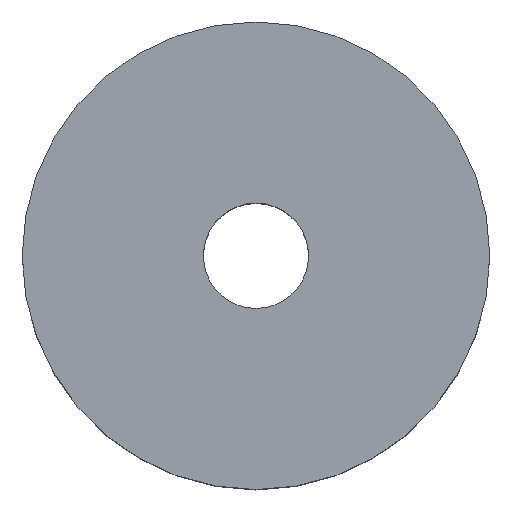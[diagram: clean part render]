
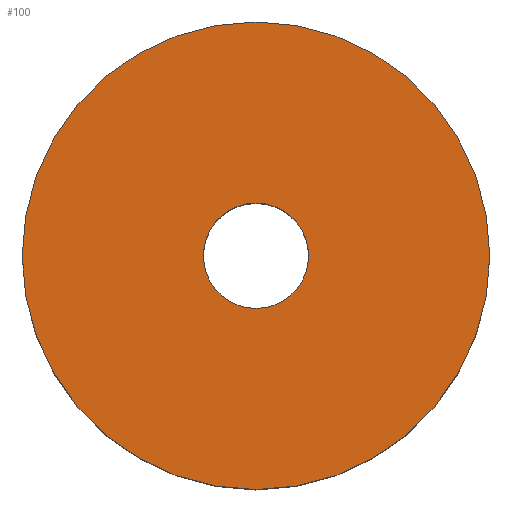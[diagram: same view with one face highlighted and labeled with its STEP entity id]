
A CAD part, top view. The second image highlights one B-rep face of the part: STEP entity #100.
In plain terms, the highlighted planar face has unit normal (0, 0, 1).
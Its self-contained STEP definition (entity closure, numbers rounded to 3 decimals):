
#5 = DIRECTION ( 'NONE',  ( 1., 0., 0. ) ) ;
#6 = DIRECTION ( 'NONE',  ( 0., 0., 1. ) ) ;
#7 = CARTESIAN_POINT ( 'NONE',  ( 0., 0., 5. ) ) ;
#12 = DIRECTION ( 'NONE',  ( 1., 0., 0. ) ) ;
#17 = VERTEX_POINT ( 'NONE', #87 ) ;
#21 = DIRECTION ( 'NONE',  ( 0., 0., 1. ) ) ;
#31 = CARTESIAN_POINT ( 'NONE',  ( 0., 0., 5. ) ) ;
#38 = CARTESIAN_POINT ( 'NONE',  ( -1.125, 0., 5. ) ) ;
#43 = CARTESIAN_POINT ( 'NONE',  ( 5., 0., 5. ) ) ;
#44 = CARTESIAN_POINT ( 'NONE',  ( -5., 0., 5. ) ) ;
#51 = DIRECTION ( 'NONE',  ( 1., 0., 0. ) ) ;
#53 = DIRECTION ( 'NONE',  ( 1., 0., 0. ) ) ;
#55 = PLANE ( 'NONE',  #179 ) ;
#59 = DIRECTION ( 'NONE',  ( 0., 0., 1. ) ) ;
#60 = CARTESIAN_POINT ( 'NONE',  ( 0., 0., 5. ) ) ;
#64 = CARTESIAN_POINT ( 'NONE',  ( 0., 0., 5. ) ) ;
#70 = DIRECTION ( 'NONE',  ( 0., 0., 1. ) ) ;
#87 = CARTESIAN_POINT ( 'NONE',  ( 1.125, 0., 5. ) ) ;
#94 = DIRECTION ( 'NONE',  ( 1., 0., 0. ) ) ;
#100 = ADVANCED_FACE ( 'NONE', ( #135, #122 ), #55, .T. ) ;
#108 = CIRCLE ( 'NONE', #161, 5. ) ;
#110 = CIRCLE ( 'NONE', #164, 1.125 ) ;
#112 = CIRCLE ( 'NONE', #171, 1.125 ) ;
#122 = FACE_OUTER_BOUND ( 'NONE', #205, .T. ) ;
#123 = CARTESIAN_POINT ( 'NONE',  ( 0., 0., 5. ) ) ;
#125 = CIRCLE ( 'NONE', #192, 5. ) ;
#135 = FACE_BOUND ( 'NONE', #149, .T. ) ;
#143 = VERTEX_POINT ( 'NONE', #44 ) ;
#146 = ORIENTED_EDGE ( 'NONE', *, *, #206, .F. ) ;
#149 = EDGE_LOOP ( 'NONE', ( #163, #146 ) ) ;
#161 = AXIS2_PLACEMENT_3D ( 'NONE', #60, #59, #51 ) ;
#163 = ORIENTED_EDGE ( 'NONE', *, *, #202, .F. ) ;
#164 = AXIS2_PLACEMENT_3D ( 'NONE', #123, #173, #94 ) ;
#171 = AXIS2_PLACEMENT_3D ( 'NONE', #31, #21, #12 ) ;
#173 = DIRECTION ( 'NONE',  ( 0., 0., 1. ) ) ;
#179 = AXIS2_PLACEMENT_3D ( 'NONE', #64, #70, #53 ) ;
#180 = ORIENTED_EDGE ( 'NONE', *, *, #200, .T. ) ;
#190 = VERTEX_POINT ( 'NONE', #43 ) ;
#192 = AXIS2_PLACEMENT_3D ( 'NONE', #7, #6, #5 ) ;
#200 = EDGE_CURVE ( 'NONE', #143, #190, #125, .T. ) ;
#202 = EDGE_CURVE ( 'NONE', #17, #213, #112, .T. ) ;
#205 = EDGE_LOOP ( 'NONE', ( #180, #211 ) ) ;
#206 = EDGE_CURVE ( 'NONE', #213, #17, #110, .T. ) ;
#208 = EDGE_CURVE ( 'NONE', #190, #143, #108, .T. ) ;
#211 = ORIENTED_EDGE ( 'NONE', *, *, #208, .T. ) ;
#213 = VERTEX_POINT ( 'NONE', #38 ) ;
